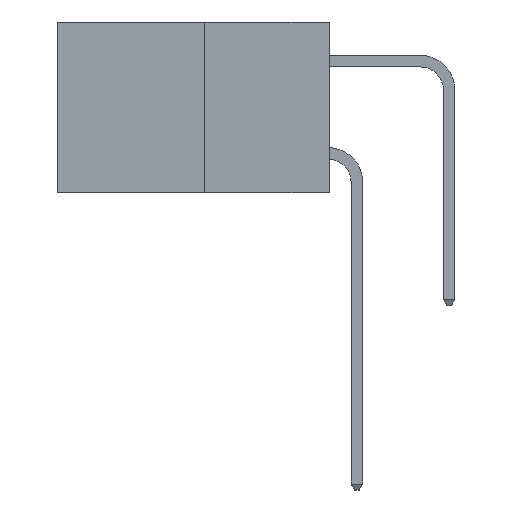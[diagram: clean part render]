
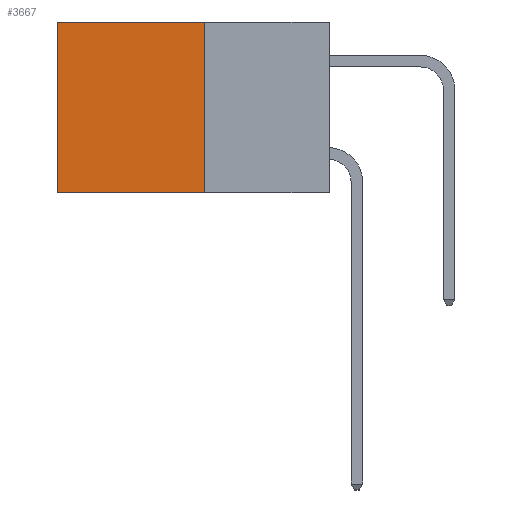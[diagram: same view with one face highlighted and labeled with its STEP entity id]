
A CAD part, left-side view. The second image highlights one B-rep face of the part: STEP entity #3667.
In plain terms, the highlighted planar face has unit normal (-1, 0, 0).
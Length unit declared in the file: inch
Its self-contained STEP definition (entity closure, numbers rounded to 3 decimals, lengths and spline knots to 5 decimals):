
#929 = VECTOR ( 'NONE', #10111, 39.37008 ) ;
#2232 = EDGE_CURVE ( 'NONE', #9085, #3549, #2964, .T. ) ;
#2415 = DIRECTION ( 'NONE',  ( 0., 0., -1. ) ) ;
#2964 = LINE ( 'NONE', #16715, #18430 ) ;
#3549 = VERTEX_POINT ( 'NONE', #3670 ) ;
#3616 = CARTESIAN_POINT ( 'NONE',  ( 0.277, 0.27, 0. ) ) ;
#3667 = ADVANCED_FACE ( 'NONE', ( #14636 ), #5877, .F. ) ;
#3670 = CARTESIAN_POINT ( 'NONE',  ( 0.277, 0.59, -0.37 ) ) ;
#4385 = EDGE_LOOP ( 'NONE', ( #12482, #14058, #7771, #7617 ) ) ;
#4927 = LINE ( 'NONE', #8559, #929 ) ;
#5060 = EDGE_CURVE ( 'NONE', #11730, #9085, #7013, .T. ) ;
#5821 = EDGE_CURVE ( 'NONE', #9693, #3549, #17034, .T. ) ;
#5877 = PLANE ( 'NONE',  #12902 ) ;
#6385 = DIRECTION ( 'NONE',  ( 1., 0., 0. ) ) ;
#6401 = DIRECTION ( 'NONE',  ( 0., 0., -1. ) ) ;
#6672 = CARTESIAN_POINT ( 'NONE',  ( 0.277, 0.27, -0.37 ) ) ;
#6774 = EDGE_CURVE ( 'NONE', #11730, #9693, #4927, .T. ) ;
#7013 = LINE ( 'NONE', #13145, #18128 ) ;
#7617 = ORIENTED_EDGE ( 'NONE', *, *, #6774, .T. ) ;
#7771 = ORIENTED_EDGE ( 'NONE', *, *, #5060, .F. ) ;
#8559 = CARTESIAN_POINT ( 'NONE',  ( 0.277, 0.27, 0. ) ) ;
#9085 = VERTEX_POINT ( 'NONE', #15610 ) ;
#9693 = VERTEX_POINT ( 'NONE', #12440 ) ;
#10111 = DIRECTION ( 'NONE',  ( 0., 1., 0. ) ) ;
#10684 = DIRECTION ( 'NONE',  ( 0., 1., 0. ) ) ;
#11730 = VERTEX_POINT ( 'NONE', #3616 ) ;
#12440 = CARTESIAN_POINT ( 'NONE',  ( 0.277, 0.59, 0. ) ) ;
#12482 = ORIENTED_EDGE ( 'NONE', *, *, #5821, .T. ) ;
#12902 = AXIS2_PLACEMENT_3D ( 'NONE', #6672, #6385, #6401 ) ;
#13145 = CARTESIAN_POINT ( 'NONE',  ( 0.277, 0.27, -0.37 ) ) ;
#14058 = ORIENTED_EDGE ( 'NONE', *, *, #2232, .F. ) ;
#14636 = FACE_OUTER_BOUND ( 'NONE', #4385, .T. ) ;
#15610 = CARTESIAN_POINT ( 'NONE',  ( 0.277, 0.27, -0.37 ) ) ;
#16587 = VECTOR ( 'NONE', #2415, 39.37008 ) ;
#16715 = CARTESIAN_POINT ( 'NONE',  ( 0.277, 0.27, -0.37 ) ) ;
#16826 = DIRECTION ( 'NONE',  ( 0., 0., -1. ) ) ;
#17034 = LINE ( 'NONE', #17322, #16587 ) ;
#17322 = CARTESIAN_POINT ( 'NONE',  ( 0.277, 0.59, -0.37 ) ) ;
#18128 = VECTOR ( 'NONE', #16826, 39.37008 ) ;
#18430 = VECTOR ( 'NONE', #10684, 39.37008 ) ;
